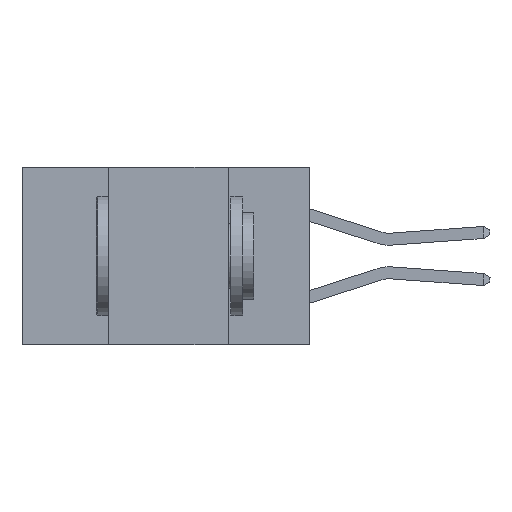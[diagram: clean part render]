
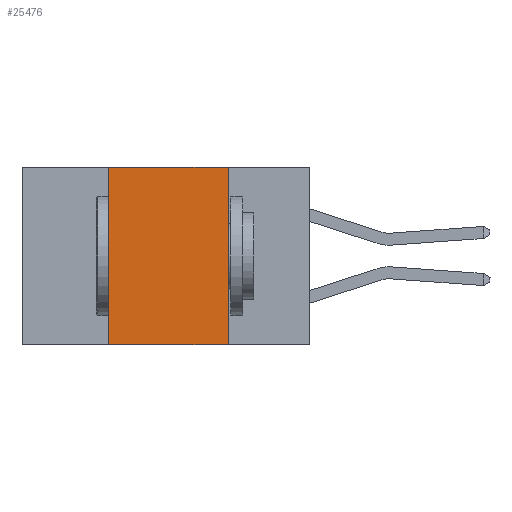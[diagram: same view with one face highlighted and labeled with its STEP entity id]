
A CAD part, left-side view. The second image highlights one B-rep face of the part: STEP entity #25476.
In plain terms, the highlighted planar face has unit normal (-1, 0, 0).
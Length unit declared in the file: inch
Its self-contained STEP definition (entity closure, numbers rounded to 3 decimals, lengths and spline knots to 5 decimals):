
#15 = CARTESIAN_POINT ( 'NONE',  ( 0., 0.42, 0. ) ) ;
#17 = DIRECTION ( 'NONE',  ( 1., 0., 0. ) ) ;
#385 = ORIENTED_EDGE ( 'NONE', *, *, #14969, .F. ) ;
#705 = CARTESIAN_POINT ( 'NONE',  ( 0., 0.42, -0.37 ) ) ;
#1616 = VECTOR ( 'NONE', #2798, 39.37008 ) ;
#2237 = LINE ( 'NONE', #4956, #24367 ) ;
#2685 = VECTOR ( 'NONE', #21464, 39.37008 ) ;
#2773 = DIRECTION ( 'NONE',  ( 0., -1., 0. ) ) ;
#2798 = DIRECTION ( 'NONE',  ( 0., 0., 1. ) ) ;
#3020 = LINE ( 'NONE', #9143, #19049 ) ;
#3535 = CARTESIAN_POINT ( 'NONE',  ( 0., 0.17, 0. ) ) ;
#3663 = VERTEX_POINT ( 'NONE', #15 ) ;
#4956 = CARTESIAN_POINT ( 'NONE',  ( 0., 0.6, -0.37 ) ) ;
#8418 = CARTESIAN_POINT ( 'NONE',  ( 0., 0.6, 0. ) ) ;
#8831 = VERTEX_POINT ( 'NONE', #16585 ) ;
#9143 = CARTESIAN_POINT ( 'NONE',  ( 0., 0.6, 0. ) ) ;
#10268 = ORIENTED_EDGE ( 'NONE', *, *, #16377, .F. ) ;
#11566 = ORIENTED_EDGE ( 'NONE', *, *, #12230, .F. ) ;
#12230 = EDGE_CURVE ( 'NONE', #24560, #8831, #13841, .T. ) ;
#12406 = EDGE_LOOP ( 'NONE', ( #11566, #385, #10268, #20661 ) ) ;
#12595 = PLANE ( 'NONE',  #13290 ) ;
#12805 = LINE ( 'NONE', #705, #1616 ) ;
#13290 = AXIS2_PLACEMENT_3D ( 'NONE', #8418, #17, #14645 ) ;
#13841 = LINE ( 'NONE', #19382, #2685 ) ;
#14645 = DIRECTION ( 'NONE',  ( 0., 0., -1. ) ) ;
#14969 = EDGE_CURVE ( 'NONE', #3663, #24560, #3020, .T. ) ;
#16377 = EDGE_CURVE ( 'NONE', #24744, #3663, #12805, .T. ) ;
#16585 = CARTESIAN_POINT ( 'NONE',  ( 0., 0.17, -0.37 ) ) ;
#17749 = EDGE_CURVE ( 'NONE', #24744, #8831, #2237, .T. ) ;
#19049 = VECTOR ( 'NONE', #2773, 39.37008 ) ;
#19382 = CARTESIAN_POINT ( 'NONE',  ( 0., 0.17, -0.37 ) ) ;
#20661 = ORIENTED_EDGE ( 'NONE', *, *, #17749, .T. ) ;
#20807 = CARTESIAN_POINT ( 'NONE',  ( 0., 0.42, -0.37 ) ) ;
#21464 = DIRECTION ( 'NONE',  ( 0., 0., -1. ) ) ;
#21568 = DIRECTION ( 'NONE',  ( 0., -1., 0. ) ) ;
#24367 = VECTOR ( 'NONE', #21568, 39.37008 ) ;
#24560 = VERTEX_POINT ( 'NONE', #3535 ) ;
#24744 = VERTEX_POINT ( 'NONE', #20807 ) ;
#25476 = ADVANCED_FACE ( 'NONE', ( #26793 ), #12595, .F. ) ;
#26793 = FACE_OUTER_BOUND ( 'NONE', #12406, .T. ) ;
